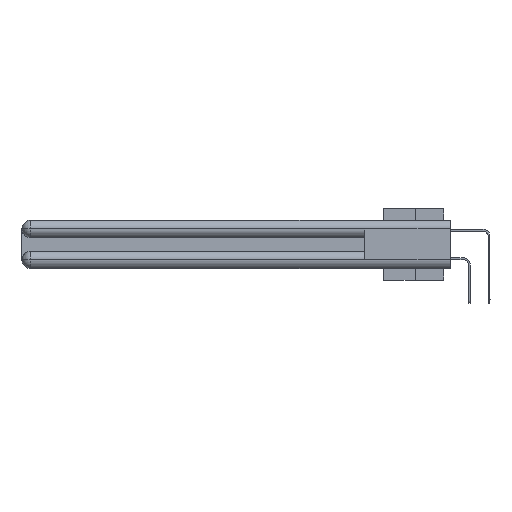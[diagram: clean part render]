
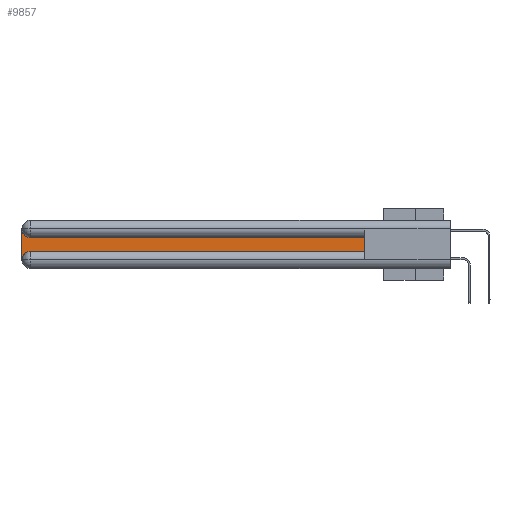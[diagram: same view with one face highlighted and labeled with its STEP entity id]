
A CAD part, left-side view. The second image highlights one B-rep face of the part: STEP entity #9857.
In plain terms, the highlighted planar face has unit normal (-1, 0, 0).
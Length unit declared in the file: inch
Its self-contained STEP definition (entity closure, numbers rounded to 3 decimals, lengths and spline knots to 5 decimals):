
#431 = EDGE_LOOP ( 'NONE', ( #23561, #3354, #19683, #613, #9496, #9710 ) ) ;
#613 = ORIENTED_EDGE ( 'NONE', *, *, #14413, .T. ) ;
#1552 = CARTESIAN_POINT ( 'NONE',  ( 0.075, 2.94, -0.0625 ) ) ;
#1627 = VERTEX_POINT ( 'NONE', #16173 ) ;
#1875 = CARTESIAN_POINT ( 'NONE',  ( 0.075, 0.6, -0.2175 ) ) ;
#2049 = LINE ( 'NONE', #13922, #17096 ) ;
#2272 = DIRECTION ( 'NONE',  ( 1., 0., 0. ) ) ;
#3036 = VECTOR ( 'NONE', #19474, 39.37008 ) ;
#3354 = ORIENTED_EDGE ( 'NONE', *, *, #9675, .T. ) ;
#3949 = CIRCLE ( 'NONE', #17607, 0.06 ) ;
#4286 = CARTESIAN_POINT ( 'NONE',  ( 0.075, 3., -0.2775 ) ) ;
#4866 = LINE ( 'NONE', #7615, #3036 ) ;
#5633 = CARTESIAN_POINT ( 'NONE',  ( 0.075, 3., -0.1225 ) ) ;
#6978 = VERTEX_POINT ( 'NONE', #22896 ) ;
#7602 = DIRECTION ( 'NONE',  ( 1., 0., 0. ) ) ;
#7615 = CARTESIAN_POINT ( 'NONE',  ( 0.075, 0.6, -0.2175 ) ) ;
#9496 = ORIENTED_EDGE ( 'NONE', *, *, #23689, .T. ) ;
#9533 = VERTEX_POINT ( 'NONE', #4286 ) ;
#9675 = EDGE_CURVE ( 'NONE', #27401, #1627, #15976, .T. ) ;
#9710 = ORIENTED_EDGE ( 'NONE', *, *, #27053, .T. ) ;
#9857 = ADVANCED_FACE ( 'NONE', ( #32611 ), #23890, .F. ) ;
#12633 = CARTESIAN_POINT ( 'NONE',  ( 0.075, 0.6, -0.2175 ) ) ;
#13572 = DIRECTION ( 'NONE',  ( 0., 0., -1. ) ) ;
#13922 = CARTESIAN_POINT ( 'NONE',  ( 0.075, 0.6, -0.1225 ) ) ;
#14413 = EDGE_CURVE ( 'NONE', #9533, #35446, #3949, .T. ) ;
#14530 = DIRECTION ( 'NONE',  ( 0., 0., -1. ) ) ;
#15976 = CIRCLE ( 'NONE', #37659, 0.06 ) ;
#16173 = CARTESIAN_POINT ( 'NONE',  ( 0.075, 3., -0.0625 ) ) ;
#16290 = LINE ( 'NONE', #36688, #17364 ) ;
#17096 = VECTOR ( 'NONE', #20861, 39.37008 ) ;
#17364 = VECTOR ( 'NONE', #13572, 39.37008 ) ;
#17607 = AXIS2_PLACEMENT_3D ( 'NONE', #29668, #2272, #14530 ) ;
#19171 = VECTOR ( 'NONE', #19390, 39.37008 ) ;
#19390 = DIRECTION ( 'NONE',  ( 0., 0., 1. ) ) ;
#19474 = DIRECTION ( 'NONE',  ( 0., -1., 0. ) ) ;
#19683 = ORIENTED_EDGE ( 'NONE', *, *, #28294, .T. ) ;
#20861 = DIRECTION ( 'NONE',  ( 0., 1., 0. ) ) ;
#22486 = CARTESIAN_POINT ( 'NONE',  ( 0.075, 2.94, -0.2175 ) ) ;
#22602 = VERTEX_POINT ( 'NONE', #12633 ) ;
#22896 = CARTESIAN_POINT ( 'NONE',  ( 0.075, 0.6, -0.1225 ) ) ;
#22962 = DIRECTION ( 'NONE',  ( 0., 0., -1. ) ) ;
#23561 = ORIENTED_EDGE ( 'NONE', *, *, #35422, .T. ) ;
#23689 = EDGE_CURVE ( 'NONE', #35446, #22602, #4866, .T. ) ;
#23890 = PLANE ( 'NONE',  #33048 ) ;
#25980 = LINE ( 'NONE', #1875, #19171 ) ;
#27053 = EDGE_CURVE ( 'NONE', #22602, #6978, #25980, .T. ) ;
#27401 = VERTEX_POINT ( 'NONE', #35843 ) ;
#28294 = EDGE_CURVE ( 'NONE', #1627, #9533, #16290, .T. ) ;
#29668 = CARTESIAN_POINT ( 'NONE',  ( 0.075, 2.94, -0.2775 ) ) ;
#29706 = DIRECTION ( 'NONE',  ( 0., 0., -1. ) ) ;
#32043 = DIRECTION ( 'NONE',  ( 1., 0., 0. ) ) ;
#32611 = FACE_OUTER_BOUND ( 'NONE', #431, .T. ) ;
#33048 = AXIS2_PLACEMENT_3D ( 'NONE', #5633, #32043, #29706 ) ;
#35422 = EDGE_CURVE ( 'NONE', #6978, #27401, #2049, .T. ) ;
#35446 = VERTEX_POINT ( 'NONE', #22486 ) ;
#35843 = CARTESIAN_POINT ( 'NONE',  ( 0.075, 2.94, -0.1225 ) ) ;
#36688 = CARTESIAN_POINT ( 'NONE',  ( 0.075, 3., -0.2175 ) ) ;
#37659 = AXIS2_PLACEMENT_3D ( 'NONE', #1552, #7602, #22962 ) ;
